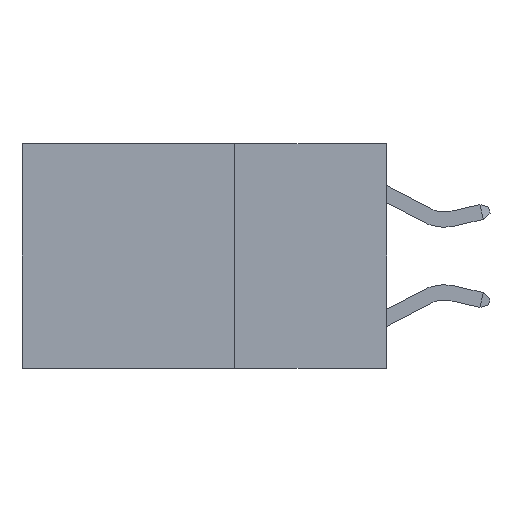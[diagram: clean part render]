
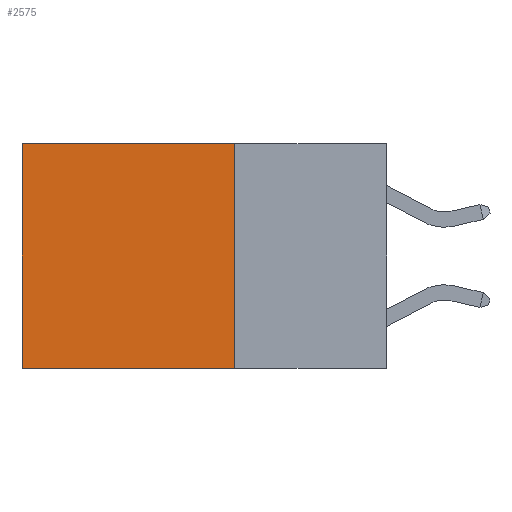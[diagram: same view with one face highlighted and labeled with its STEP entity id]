
A CAD part, left-side view. The second image highlights one B-rep face of the part: STEP entity #2575.
In plain terms, the highlighted planar face has unit normal (-1, 0, 0).
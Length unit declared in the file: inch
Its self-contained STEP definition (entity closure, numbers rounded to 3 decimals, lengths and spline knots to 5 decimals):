
#977 = DIRECTION ( 'NONE',  ( 0., 0., -1. ) ) ;
#1589 = ORIENTED_EDGE ( 'NONE', *, *, #4827, .T. ) ;
#2098 = CARTESIAN_POINT ( 'NONE',  ( 0.2625, 0.6, 0. ) ) ;
#2444 = FACE_OUTER_BOUND ( 'NONE', #7755, .T. ) ;
#2575 = ADVANCED_FACE ( 'NONE', ( #2444 ), #3242, .F. ) ;
#2817 = VERTEX_POINT ( 'NONE', #11540 ) ;
#3121 = DIRECTION ( 'NONE',  ( 0., 0., -1. ) ) ;
#3125 = DIRECTION ( 'NONE',  ( 0., 1., 0. ) ) ;
#3163 = DIRECTION ( 'NONE',  ( 1., 0., 0. ) ) ;
#3242 = PLANE ( 'NONE',  #4949 ) ;
#3259 = CARTESIAN_POINT ( 'NONE',  ( 0.2625, 0.25, 0. ) ) ;
#3773 = VERTEX_POINT ( 'NONE', #6210 ) ;
#4460 = ORIENTED_EDGE ( 'NONE', *, *, #11302, .F. ) ;
#4827 = EDGE_CURVE ( 'NONE', #3773, #2817, #10890, .T. ) ;
#4949 = AXIS2_PLACEMENT_3D ( 'NONE', #3259, #3163, #3121 ) ;
#5340 = CARTESIAN_POINT ( 'NONE',  ( 0.2625, 0.25, 0. ) ) ;
#5489 = CARTESIAN_POINT ( 'NONE',  ( 0.2625, 0.25, -0.37 ) ) ;
#5934 = VECTOR ( 'NONE', #977, 39.37008 ) ;
#6210 = CARTESIAN_POINT ( 'NONE',  ( 0.2625, 0.6, 0. ) ) ;
#6450 = VECTOR ( 'NONE', #3125, 39.37008 ) ;
#6486 = VERTEX_POINT ( 'NONE', #10977 ) ;
#6545 = VECTOR ( 'NONE', #7936, 39.37008 ) ;
#6807 = EDGE_CURVE ( 'NONE', #6486, #7681, #8285, .T. ) ;
#6955 = CARTESIAN_POINT ( 'NONE',  ( 0.2625, 0.25, 0. ) ) ;
#7681 = VERTEX_POINT ( 'NONE', #5489 ) ;
#7755 = EDGE_LOOP ( 'NONE', ( #1589, #4460, #9231, #11519 ) ) ;
#7843 = VECTOR ( 'NONE', #9741, 39.37008 ) ;
#7852 = CARTESIAN_POINT ( 'NONE',  ( 0.2625, 0.25, -0.37 ) ) ;
#7936 = DIRECTION ( 'NONE',  ( 0., 0., -1. ) ) ;
#8285 = LINE ( 'NONE', #6955, #5934 ) ;
#9231 = ORIENTED_EDGE ( 'NONE', *, *, #6807, .F. ) ;
#9741 = DIRECTION ( 'NONE',  ( 0., 1., 0. ) ) ;
#10419 = LINE ( 'NONE', #5340, #7843 ) ;
#10476 = EDGE_CURVE ( 'NONE', #6486, #3773, #10419, .T. ) ;
#10890 = LINE ( 'NONE', #2098, #6545 ) ;
#10977 = CARTESIAN_POINT ( 'NONE',  ( 0.2625, 0.25, 0. ) ) ;
#11083 = LINE ( 'NONE', #7852, #6450 ) ;
#11302 = EDGE_CURVE ( 'NONE', #7681, #2817, #11083, .T. ) ;
#11519 = ORIENTED_EDGE ( 'NONE', *, *, #10476, .T. ) ;
#11540 = CARTESIAN_POINT ( 'NONE',  ( 0.2625, 0.6, -0.37 ) ) ;
